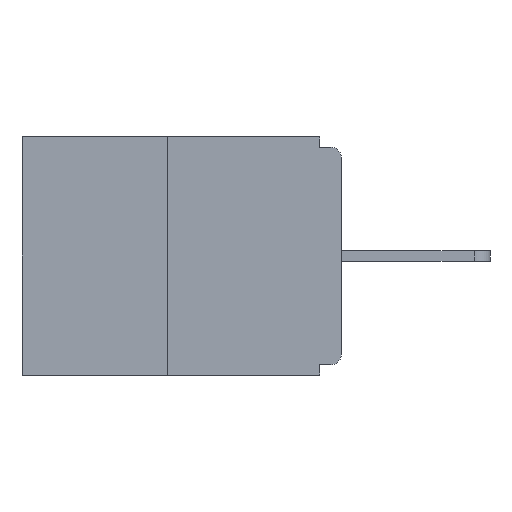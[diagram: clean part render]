
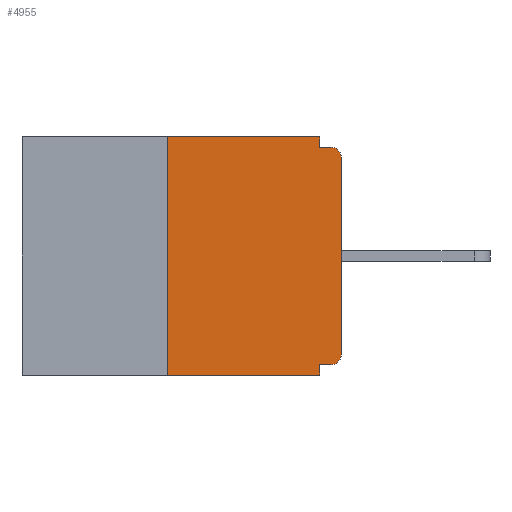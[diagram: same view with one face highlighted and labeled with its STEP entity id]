
A CAD part, left-side view. The second image highlights one B-rep face of the part: STEP entity #4955.
In plain terms, the highlighted planar face has unit normal (-1, 0, 0).
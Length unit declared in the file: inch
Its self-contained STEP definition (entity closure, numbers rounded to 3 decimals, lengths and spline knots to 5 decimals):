
#56 = ORIENTED_EDGE ( 'NONE', *, *, #17986, .T. ) ;
#78 = ORIENTED_EDGE ( 'NONE', *, *, #15041, .T. ) ;
#258 = CARTESIAN_POINT ( 'NONE',  ( 0., 0.031, 0. ) ) ;
#337 = ORIENTED_EDGE ( 'NONE', *, *, #9146, .F. ) ;
#454 = VECTOR ( 'NONE', #7676, 39.37008 ) ;
#494 = ORIENTED_EDGE ( 'NONE', *, *, #3747, .F. ) ;
#934 = EDGE_CURVE ( 'NONE', #8833, #18049, #8091, .T. ) ;
#1053 = CARTESIAN_POINT ( 'NONE',  ( 0., 0.031, 0. ) ) ;
#1173 = DIRECTION ( 'NONE',  ( 0., -1., 0. ) ) ;
#1234 = VERTEX_POINT ( 'NONE', #2152 ) ;
#1578 = DIRECTION ( 'NONE',  ( 0., 1., 0. ) ) ;
#1623 = CARTESIAN_POINT ( 'NONE',  ( 0., 0., -0.328 ) ) ;
#1661 = CARTESIAN_POINT ( 'NONE',  ( 0., 0.015, -0.313 ) ) ;
#2127 = CARTESIAN_POINT ( 'NONE',  ( 0., 0.015, -0.328 ) ) ;
#2152 = CARTESIAN_POINT ( 'NONE',  ( 0., 0.031, -0.343 ) ) ;
#3203 = VERTEX_POINT ( 'NONE', #5265 ) ;
#3333 = EDGE_CURVE ( 'NONE', #14450, #3203, #16051, .T. ) ;
#3427 = DIRECTION ( 'NONE',  ( 0., 0., -1. ) ) ;
#3665 = VECTOR ( 'NONE', #1578, 39.37008 ) ;
#3747 = EDGE_CURVE ( 'NONE', #10605, #14789, #5073, .T. ) ;
#3861 = LINE ( 'NONE', #19658, #20396 ) ;
#4482 = VECTOR ( 'NONE', #8101, 39.37008 ) ;
#4529 = LINE ( 'NONE', #7250, #12197 ) ;
#4673 = VERTEX_POINT ( 'NONE', #15566 ) ;
#4775 = CARTESIAN_POINT ( 'NONE',  ( 0., 0.46, 0. ) ) ;
#4955 = ADVANCED_FACE ( 'NONE', ( #12210 ), #20139, .F. ) ;
#5073 = LINE ( 'NONE', #1053, #454 ) ;
#5265 = CARTESIAN_POINT ( 'NONE',  ( 0., 0.25, 0. ) ) ;
#5364 = CARTESIAN_POINT ( 'NONE',  ( 0., 0.031, -0.328 ) ) ;
#6275 = ORIENTED_EDGE ( 'NONE', *, *, #15757, .T. ) ;
#6462 = AXIS2_PLACEMENT_3D ( 'NONE', #1661, #13260, #3427 ) ;
#6682 = VERTEX_POINT ( 'NONE', #16958 ) ;
#6804 = AXIS2_PLACEMENT_3D ( 'NONE', #10054, #21017, #11656 ) ;
#6817 = CARTESIAN_POINT ( 'NONE',  ( 0., 0.25, -0.343 ) ) ;
#6859 = CIRCLE ( 'NONE', #6462, 0.015 ) ;
#7250 = CARTESIAN_POINT ( 'NONE',  ( 0., 0.031, -0.343 ) ) ;
#7289 = ORIENTED_EDGE ( 'NONE', *, *, #19845, .T. ) ;
#7676 = DIRECTION ( 'NONE',  ( 0., 0., -1. ) ) ;
#7984 = VECTOR ( 'NONE', #20662, 39.37008 ) ;
#8091 = LINE ( 'NONE', #1623, #3665 ) ;
#8101 = DIRECTION ( 'NONE',  ( 0., -1., 0. ) ) ;
#8496 = VECTOR ( 'NONE', #1173, 39.37008 ) ;
#8833 = VERTEX_POINT ( 'NONE', #2127 ) ;
#9146 = EDGE_CURVE ( 'NONE', #14789, #6682, #12790, .T. ) ;
#9332 = CARTESIAN_POINT ( 'NONE',  ( 0., 0.031, -0.015 ) ) ;
#10054 = CARTESIAN_POINT ( 'NONE',  ( 0., 0.015, -0.03 ) ) ;
#10605 = VERTEX_POINT ( 'NONE', #258 ) ;
#11141 = ORIENTED_EDGE ( 'NONE', *, *, #12553, .F. ) ;
#11410 = CARTESIAN_POINT ( 'NONE',  ( 0., 0., -0.03 ) ) ;
#11656 = DIRECTION ( 'NONE',  ( 0., 0., -1. ) ) ;
#12197 = VECTOR ( 'NONE', #13792, 39.37008 ) ;
#12210 = FACE_OUTER_BOUND ( 'NONE', #19792, .T. ) ;
#12553 = EDGE_CURVE ( 'NONE', #18049, #1234, #4529, .T. ) ;
#12790 = LINE ( 'NONE', #20567, #8496 ) ;
#13260 = DIRECTION ( 'NONE',  ( -1., 0., 0. ) ) ;
#13302 = CARTESIAN_POINT ( 'NONE',  ( 0., 0., 0. ) ) ;
#13792 = DIRECTION ( 'NONE',  ( 0., 0., -1. ) ) ;
#14345 = VERTEX_POINT ( 'NONE', #11410 ) ;
#14450 = VERTEX_POINT ( 'NONE', #6817 ) ;
#14789 = VERTEX_POINT ( 'NONE', #9332 ) ;
#15041 = EDGE_CURVE ( 'NONE', #14345, #6682, #17550, .T. ) ;
#15566 = CARTESIAN_POINT ( 'NONE',  ( 0., 0., -0.313 ) ) ;
#15757 = EDGE_CURVE ( 'NONE', #14450, #1234, #3861, .T. ) ;
#15818 = LINE ( 'NONE', #13302, #19419 ) ;
#16051 = LINE ( 'NONE', #21047, #7984 ) ;
#16654 = DIRECTION ( 'NONE',  ( 0., -1., 0. ) ) ;
#16958 = CARTESIAN_POINT ( 'NONE',  ( 0., 0.015, -0.015 ) ) ;
#17550 = CIRCLE ( 'NONE', #6804, 0.015 ) ;
#17562 = ORIENTED_EDGE ( 'NONE', *, *, #20922, .F. ) ;
#17842 = LINE ( 'NONE', #4775, #4482 ) ;
#17947 = DIRECTION ( 'NONE',  ( 0., 0., 1. ) ) ;
#17986 = EDGE_CURVE ( 'NONE', #4673, #14345, #15818, .T. ) ;
#18049 = VERTEX_POINT ( 'NONE', #5364 ) ;
#18521 = ORIENTED_EDGE ( 'NONE', *, *, #3333, .F. ) ;
#19419 = VECTOR ( 'NONE', #17947, 39.37008 ) ;
#19500 = ORIENTED_EDGE ( 'NONE', *, *, #934, .F. ) ;
#19658 = CARTESIAN_POINT ( 'NONE',  ( 0., 0.46, -0.343 ) ) ;
#19792 = EDGE_LOOP ( 'NONE', ( #17562, #18521, #6275, #11141, #19500, #7289, #56, #78, #337, #494 ) ) ;
#19845 = EDGE_CURVE ( 'NONE', #8833, #4673, #6859, .T. ) ;
#20030 = CARTESIAN_POINT ( 'NONE',  ( 0., 0.46, 0. ) ) ;
#20131 = DIRECTION ( 'NONE',  ( 0., 0., -1. ) ) ;
#20139 = PLANE ( 'NONE',  #20761 ) ;
#20396 = VECTOR ( 'NONE', #16654, 39.37008 ) ;
#20567 = CARTESIAN_POINT ( 'NONE',  ( 0., 0., -0.015 ) ) ;
#20662 = DIRECTION ( 'NONE',  ( 0., 0., 1. ) ) ;
#20761 = AXIS2_PLACEMENT_3D ( 'NONE', #20030, #20873, #20131 ) ;
#20873 = DIRECTION ( 'NONE',  ( 1., 0., 0. ) ) ;
#20922 = EDGE_CURVE ( 'NONE', #3203, #10605, #17842, .T. ) ;
#21017 = DIRECTION ( 'NONE',  ( -1., 0., 0. ) ) ;
#21047 = CARTESIAN_POINT ( 'NONE',  ( 0., 0.25, 0. ) ) ;
